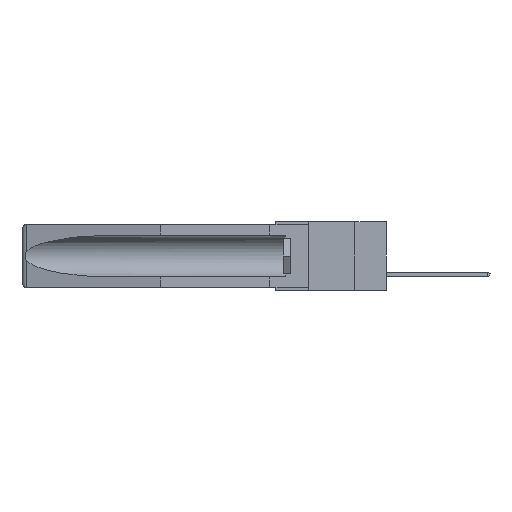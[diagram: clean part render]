
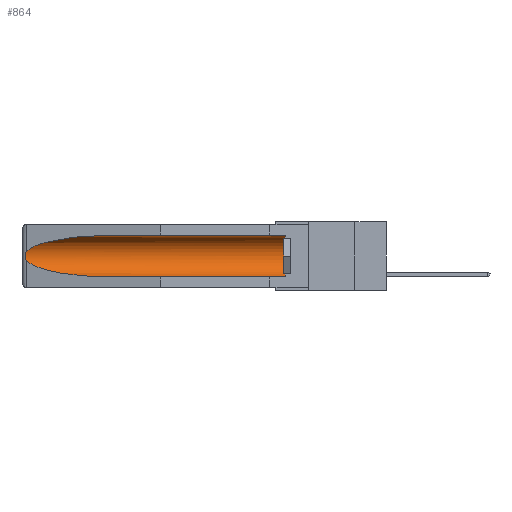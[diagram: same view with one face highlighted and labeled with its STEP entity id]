
A CAD part, left-side view. The second image highlights one B-rep face of the part: STEP entity #864.
In plain terms, the highlighted cylindrical face has radius 2.857 mm (diameter 5.715 mm), a partial arc.
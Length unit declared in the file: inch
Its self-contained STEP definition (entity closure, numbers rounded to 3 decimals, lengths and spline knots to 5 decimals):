
#2 = CARTESIAN_POINT ( 'NONE',  ( 0.26655, 1.53094, -0.18657 ) ) ;
#86 = CARTESIAN_POINT ( 'NONE',  ( 0.21114, 1.30732, -0.059 ) ) ;
#198 = CARTESIAN_POINT ( 'NONE',  ( 0.26537, 1.52718, -0.14972 ) ) ;
#256 = ORIENTED_EDGE ( 'NONE', *, *, #6075, .T. ) ;
#433 = ORIENTED_EDGE ( 'NONE', *, *, #16750, .F. ) ;
#699 = CARTESIAN_POINT ( 'NONE',  ( 0.26537, 1.52718, -0.19328 ) ) ;
#864 = ADVANCED_FACE ( 'NONE', ( #9554 ), #1694, .F. ) ;
#1028 = EDGE_CURVE ( 'NONE', #4318, #12824, #7394, .T. ) ;
#1154 = AXIS2_PLACEMENT_3D ( 'NONE', #12166, #3108, #19634 ) ;
#1632 = CARTESIAN_POINT ( 'NONE',  ( 0.25451, 1.48313, -0.09465 ) ) ;
#1694 = CYLINDRICAL_SURFACE ( 'NONE', #8307, 0.1125 ) ;
#3108 = DIRECTION ( 'NONE',  ( 0., -1., 0. ) ) ;
#3459 = CARTESIAN_POINT ( 'NONE',  ( 0.155, 0.126, -0.059 ) ) ;
#3670 = ORIENTED_EDGE ( 'NONE', *, *, #14585, .T. ) ;
#3775 =( BOUNDED_CURVE ( )  B_SPLINE_CURVE ( 3, ( #17049, #13975, #9415, #9348 ),
 .UNSPECIFIED., .F., .F. ) 
 B_SPLINE_CURVE_WITH_KNOTS ( ( 4, 4 ),
 ( 0.1948, 1.5708 ),
 .UNSPECIFIED. ) 
 CURVE ( )  GEOMETRIC_REPRESENTATION_ITEM ( )  RATIONAL_B_SPLINE_CURVE ( ( 1., 0.848, 0.848, 1. ) ) 
 REPRESENTATION_ITEM ( '' )  );
#4291 = EDGE_LOOP ( 'NONE', ( #12573, #14832, #3670, #433, #15600, #256 ) ) ;
#4318 = VERTEX_POINT ( 'NONE', #13652 ) ;
#4395 = B_SPLINE_CURVE_WITH_KNOTS ( 'NONE', 3,
 ( #198, #16764, #16827, #12086, #6183, #6108, #7679, #2, #12345, #16692 ),
 .UNSPECIFIED., .F., .F.,
 ( 4, 2, 2, 2, 4 ),
 ( 0., 0.00029, 0.00058, 0.00087, 0.00117 ),
 .UNSPECIFIED. ) ;
#5150 = DIRECTION ( 'NONE',  ( 0., 0., 1. ) ) ;
#6029 = CARTESIAN_POINT ( 'NONE',  ( 0.155, 1.07973, -0.059 ) ) ;
#6075 = EDGE_CURVE ( 'NONE', #12824, #11956, #17986, .T. ) ;
#6108 = CARTESIAN_POINT ( 'NONE',  ( 0.2675, 1.53308, -0.17534 ) ) ;
#6183 = CARTESIAN_POINT ( 'NONE',  ( 0.2675, 1.53308, -0.16763 ) ) ;
#6860 = VERTEX_POINT ( 'NONE', #699 ) ;
#7259 = DIRECTION ( 'NONE',  ( 0., 1., 0. ) ) ;
#7394 = CIRCLE ( 'NONE', #1154, 0.1125 ) ;
#7679 = CARTESIAN_POINT ( 'NONE',  ( 0.2673, 1.53269, -0.17917 ) ) ;
#8307 = AXIS2_PLACEMENT_3D ( 'NONE', #11158, #12803, #5150 ) ;
#8440 = EDGE_CURVE ( 'NONE', #11956, #15552, #16431, .T. ) ;
#8467 = DIRECTION ( 'NONE',  ( 0., 1., 0. ) ) ;
#8474 = VECTOR ( 'NONE', #8467, 39.37008 ) ;
#9348 = CARTESIAN_POINT ( 'NONE',  ( 0.155, 1.07973, -0.284 ) ) ;
#9415 = CARTESIAN_POINT ( 'NONE',  ( 0.21114, 1.30732, -0.284 ) ) ;
#9554 = FACE_OUTER_BOUND ( 'NONE', #4291, .T. ) ;
#10020 = VERTEX_POINT ( 'NONE', #14842 ) ;
#11158 = CARTESIAN_POINT ( 'NONE',  ( 0.155, -0.30754, -0.1715 ) ) ;
#11956 = VERTEX_POINT ( 'NONE', #6029 ) ;
#12086 = CARTESIAN_POINT ( 'NONE',  ( 0.2673, 1.5327, -0.16383 ) ) ;
#12166 = CARTESIAN_POINT ( 'NONE',  ( 0.155, 0.126, -0.1715 ) ) ;
#12227 = CARTESIAN_POINT ( 'NONE',  ( 0.26537, 1.52718, -0.14972 ) ) ;
#12345 = CARTESIAN_POINT ( 'NONE',  ( 0.26597, 1.5296, -0.19026 ) ) ;
#12408 = CARTESIAN_POINT ( 'NONE',  ( 0.26537, 1.52718, -0.14972 ) ) ;
#12573 = ORIENTED_EDGE ( 'NONE', *, *, #8440, .T. ) ;
#12803 = DIRECTION ( 'NONE',  ( 0., 1., 0. ) ) ;
#12824 = VERTEX_POINT ( 'NONE', #3459 ) ;
#13652 = CARTESIAN_POINT ( 'NONE',  ( 0.155, 0.126, -0.284 ) ) ;
#13975 = CARTESIAN_POINT ( 'NONE',  ( 0.25451, 1.48313, -0.24835 ) ) ;
#14585 = EDGE_CURVE ( 'NONE', #6860, #10020, #3775, .T. ) ;
#14832 = ORIENTED_EDGE ( 'NONE', *, *, #18310, .T. ) ;
#14842 = CARTESIAN_POINT ( 'NONE',  ( 0.155, 1.07973, -0.284 ) ) ;
#14865 = CARTESIAN_POINT ( 'NONE',  ( 0.155, -0.30754, -0.284 ) ) ;
#15552 = VERTEX_POINT ( 'NONE', #12408 ) ;
#15600 = ORIENTED_EDGE ( 'NONE', *, *, #1028, .T. ) ;
#16431 =( BOUNDED_CURVE ( )  B_SPLINE_CURVE ( 3, ( #16570, #86, #1632, #12227 ),
 .UNSPECIFIED., .F., .F. ) 
 B_SPLINE_CURVE_WITH_KNOTS ( ( 4, 4 ),
 ( 4.71239, 6.08839 ),
 .UNSPECIFIED. ) 
 CURVE ( )  GEOMETRIC_REPRESENTATION_ITEM ( )  RATIONAL_B_SPLINE_CURVE ( ( 1., 0.848, 0.848, 1. ) ) 
 REPRESENTATION_ITEM ( '' )  );
#16505 = VECTOR ( 'NONE', #7259, 39.37008 ) ;
#16570 = CARTESIAN_POINT ( 'NONE',  ( 0.155, 1.07973, -0.059 ) ) ;
#16692 = CARTESIAN_POINT ( 'NONE',  ( 0.26537, 1.52718, -0.19328 ) ) ;
#16750 = EDGE_CURVE ( 'NONE', #4318, #10020, #18897, .T. ) ;
#16764 = CARTESIAN_POINT ( 'NONE',  ( 0.26597, 1.52961, -0.15275 ) ) ;
#16827 = CARTESIAN_POINT ( 'NONE',  ( 0.26654, 1.53092, -0.15636 ) ) ;
#17049 = CARTESIAN_POINT ( 'NONE',  ( 0.26537, 1.52718, -0.19328 ) ) ;
#17580 = CARTESIAN_POINT ( 'NONE',  ( 0.155, -0.30754, -0.059 ) ) ;
#17986 = LINE ( 'NONE', #17580, #8474 ) ;
#18310 = EDGE_CURVE ( 'NONE', #15552, #6860, #4395, .T. ) ;
#18897 = LINE ( 'NONE', #14865, #16505 ) ;
#19634 = DIRECTION ( 'NONE',  ( 0., 0., 1. ) ) ;
